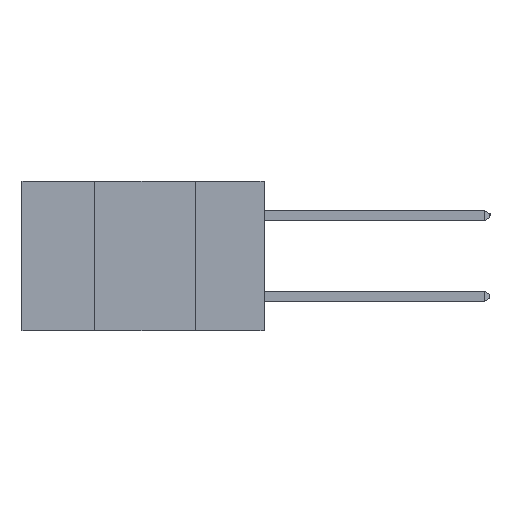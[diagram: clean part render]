
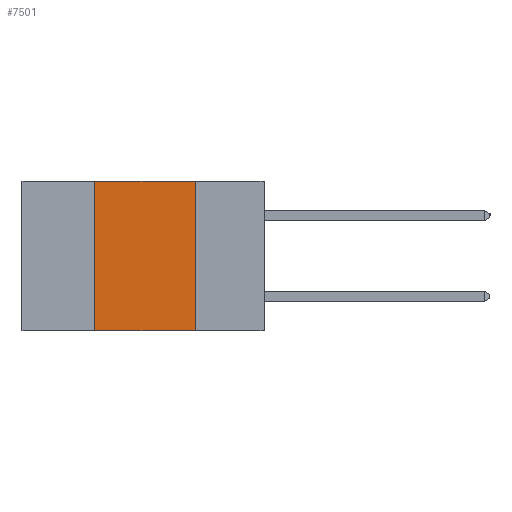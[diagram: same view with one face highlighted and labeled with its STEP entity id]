
A CAD part, left-side view. The second image highlights one B-rep face of the part: STEP entity #7501.
In plain terms, the highlighted planar face has unit normal (-1, 0, 0).
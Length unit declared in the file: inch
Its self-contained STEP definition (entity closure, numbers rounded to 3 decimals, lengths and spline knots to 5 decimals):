
#1274 = VERTEX_POINT ( 'NONE', #8012 ) ;
#2206 = CARTESIAN_POINT ( 'NONE',  ( 0., 0.42, -0.37 ) ) ;
#2302 = ORIENTED_EDGE ( 'NONE', *, *, #14429, .F. ) ;
#2860 = LINE ( 'NONE', #9840, #17041 ) ;
#2909 = LINE ( 'NONE', #4689, #6272 ) ;
#3382 = CARTESIAN_POINT ( 'NONE',  ( 0., 0.17, 0. ) ) ;
#3764 = EDGE_LOOP ( 'NONE', ( #9883, #16558, #2302, #14611 ) ) ;
#3868 = VERTEX_POINT ( 'NONE', #9073 ) ;
#4689 = CARTESIAN_POINT ( 'NONE',  ( 0., 0.6, 0. ) ) ;
#4809 = FACE_OUTER_BOUND ( 'NONE', #3764, .T. ) ;
#5813 = VECTOR ( 'NONE', #11040, 39.37008 ) ;
#6272 = VECTOR ( 'NONE', #15656, 39.37008 ) ;
#6681 = PLANE ( 'NONE',  #12967 ) ;
#7501 = ADVANCED_FACE ( 'NONE', ( #4809 ), #6681, .F. ) ;
#8012 = CARTESIAN_POINT ( 'NONE',  ( 0., 0.17, 0. ) ) ;
#8106 = DIRECTION ( 'NONE',  ( 0., 0., -1. ) ) ;
#9073 = CARTESIAN_POINT ( 'NONE',  ( 0., 0.42, 0. ) ) ;
#9543 = LINE ( 'NONE', #9690, #5813 ) ;
#9690 = CARTESIAN_POINT ( 'NONE',  ( 0., 0.6, -0.37 ) ) ;
#9840 = CARTESIAN_POINT ( 'NONE',  ( 0., 0.42, 0. ) ) ;
#9883 = ORIENTED_EDGE ( 'NONE', *, *, #16459, .F. ) ;
#10762 = CARTESIAN_POINT ( 'NONE',  ( 0., 0.6, 0. ) ) ;
#11040 = DIRECTION ( 'NONE',  ( 0., -1., 0. ) ) ;
#11189 = DIRECTION ( 'NONE',  ( 0., 0., 1. ) ) ;
#11332 = VECTOR ( 'NONE', #11747, 39.37008 ) ;
#11747 = DIRECTION ( 'NONE',  ( 0., 0., -1. ) ) ;
#12967 = AXIS2_PLACEMENT_3D ( 'NONE', #10762, #16177, #8106 ) ;
#13181 = EDGE_CURVE ( 'NONE', #13644, #14981, #9543, .T. ) ;
#13644 = VERTEX_POINT ( 'NONE', #2206 ) ;
#14429 = EDGE_CURVE ( 'NONE', #13644, #3868, #2860, .T. ) ;
#14611 = ORIENTED_EDGE ( 'NONE', *, *, #13181, .T. ) ;
#14932 = LINE ( 'NONE', #3382, #11332 ) ;
#14981 = VERTEX_POINT ( 'NONE', #17724 ) ;
#15656 = DIRECTION ( 'NONE',  ( 0., -1., 0. ) ) ;
#16177 = DIRECTION ( 'NONE',  ( 1., 0., 0. ) ) ;
#16459 = EDGE_CURVE ( 'NONE', #1274, #14981, #14932, .T. ) ;
#16558 = ORIENTED_EDGE ( 'NONE', *, *, #17635, .F. ) ;
#17041 = VECTOR ( 'NONE', #11189, 39.37008 ) ;
#17635 = EDGE_CURVE ( 'NONE', #3868, #1274, #2909, .T. ) ;
#17724 = CARTESIAN_POINT ( 'NONE',  ( 0., 0.17, -0.37 ) ) ;
